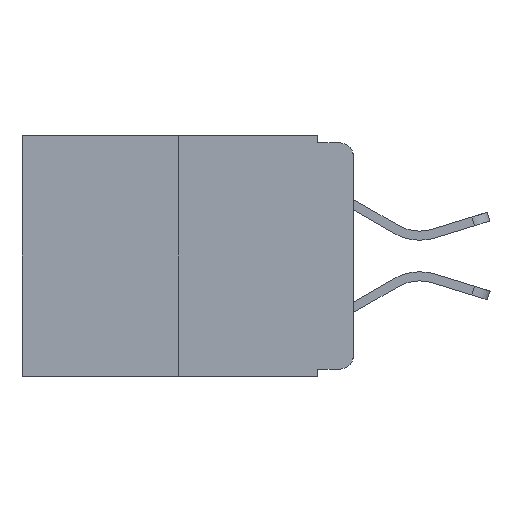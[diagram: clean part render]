
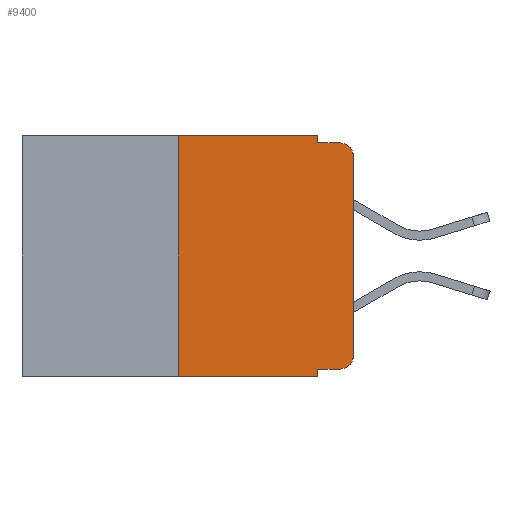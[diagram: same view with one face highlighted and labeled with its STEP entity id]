
A CAD part, left-side view. The second image highlights one B-rep face of the part: STEP entity #9400.
In plain terms, the highlighted planar face has unit normal (-1, 0, 0).
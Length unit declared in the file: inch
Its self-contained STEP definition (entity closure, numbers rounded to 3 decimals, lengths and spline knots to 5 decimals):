
#625 = LINE ( 'NONE', #13521, #10112 ) ;
#638 = EDGE_CURVE ( 'NONE', #16584, #15708, #14473, .T. ) ;
#1058 = ORIENTED_EDGE ( 'NONE', *, *, #5040, .T. ) ;
#1407 = CARTESIAN_POINT ( 'NONE',  ( 0., 0.25, 0. ) ) ;
#1543 = LINE ( 'NONE', #2735, #7409 ) ;
#1629 = ORIENTED_EDGE ( 'NONE', *, *, #3790, .T. ) ;
#2306 = CARTESIAN_POINT ( 'NONE',  ( 0., 0.051, 0. ) ) ;
#2574 = CIRCLE ( 'NONE', #13449, 0.02 ) ;
#2659 = ORIENTED_EDGE ( 'NONE', *, *, #20223, .F. ) ;
#2735 = CARTESIAN_POINT ( 'NONE',  ( 0., 0.473, -0.343 ) ) ;
#2738 = EDGE_CURVE ( 'NONE', #10975, #7517, #20059, .T. ) ;
#3047 = DIRECTION ( 'NONE',  ( 0., -1., 0. ) ) ;
#3286 = DIRECTION ( 'NONE',  ( 0., 0., -1. ) ) ;
#3416 = AXIS2_PLACEMENT_3D ( 'NONE', #12860, #17867, #3286 ) ;
#3738 = DIRECTION ( 'NONE',  ( 0., 0., 1. ) ) ;
#3790 = EDGE_CURVE ( 'NONE', #5624, #16306, #1543, .T. ) ;
#4012 = VERTEX_POINT ( 'NONE', #6872 ) ;
#4794 = CARTESIAN_POINT ( 'NONE',  ( 0., 0.051, -0.333 ) ) ;
#5040 = EDGE_CURVE ( 'NONE', #9668, #16584, #625, .T. ) ;
#5222 = VERTEX_POINT ( 'NONE', #7652 ) ;
#5250 = CARTESIAN_POINT ( 'NONE',  ( 0., 0.051, -0.01 ) ) ;
#5541 = ORIENTED_EDGE ( 'NONE', *, *, #6888, .T. ) ;
#5624 = VERTEX_POINT ( 'NONE', #10834 ) ;
#5826 = CARTESIAN_POINT ( 'NONE',  ( 0., 0., -0.313 ) ) ;
#6172 = EDGE_CURVE ( 'NONE', #5222, #15491, #6612, .T. ) ;
#6262 = EDGE_LOOP ( 'NONE', ( #1058, #16163, #14647, #13093, #2659, #13469, #1629, #20280, #6649, #5541 ) ) ;
#6320 = LINE ( 'NONE', #20997, #15250 ) ;
#6612 = LINE ( 'NONE', #11404, #10405 ) ;
#6649 = ORIENTED_EDGE ( 'NONE', *, *, #2738, .T. ) ;
#6872 = CARTESIAN_POINT ( 'NONE',  ( 0., 0.25, 0. ) ) ;
#6888 = EDGE_CURVE ( 'NONE', #7517, #9668, #2574, .T. ) ;
#7093 = EDGE_CURVE ( 'NONE', #5624, #4012, #10799, .T. ) ;
#7277 = CARTESIAN_POINT ( 'NONE',  ( 0., 0.051, -0.333 ) ) ;
#7349 = CARTESIAN_POINT ( 'NONE',  ( 0., 0.051, -0.343 ) ) ;
#7409 = VECTOR ( 'NONE', #3047, 39.37008 ) ;
#7517 = VERTEX_POINT ( 'NONE', #20351 ) ;
#7615 = LINE ( 'NONE', #2306, #19256 ) ;
#7652 = CARTESIAN_POINT ( 'NONE',  ( 0., 0.051, 0. ) ) ;
#8524 = EDGE_CURVE ( 'NONE', #15491, #15708, #10046, .T. ) ;
#9400 = ADVANCED_FACE ( 'NONE', ( #11179 ), #19464, .F. ) ;
#9668 = VERTEX_POINT ( 'NONE', #5826 ) ;
#9707 = DIRECTION ( 'NONE',  ( 0., 0., -1. ) ) ;
#10046 = LINE ( 'NONE', #5250, #10790 ) ;
#10112 = VECTOR ( 'NONE', #3738, 39.37008 ) ;
#10157 = DIRECTION ( 'NONE',  ( 0., -1., 0. ) ) ;
#10405 = VECTOR ( 'NONE', #9707, 39.37008 ) ;
#10790 = VECTOR ( 'NONE', #10157, 39.37008 ) ;
#10799 = LINE ( 'NONE', #1407, #11808 ) ;
#10834 = CARTESIAN_POINT ( 'NONE',  ( 0., 0.25, -0.343 ) ) ;
#10975 = VERTEX_POINT ( 'NONE', #4794 ) ;
#11179 = FACE_OUTER_BOUND ( 'NONE', #6262, .T. ) ;
#11404 = CARTESIAN_POINT ( 'NONE',  ( 0., 0.051, 0. ) ) ;
#11808 = VECTOR ( 'NONE', #17500, 39.37008 ) ;
#12276 = DIRECTION ( 'NONE',  ( -1., 0., 0. ) ) ;
#12368 = CARTESIAN_POINT ( 'NONE',  ( 0., 0.02, -0.03 ) ) ;
#12860 = CARTESIAN_POINT ( 'NONE',  ( 0., 0.473, 0. ) ) ;
#13093 = ORIENTED_EDGE ( 'NONE', *, *, #6172, .F. ) ;
#13449 = AXIS2_PLACEMENT_3D ( 'NONE', #20161, #12276, #20374 ) ;
#13469 = ORIENTED_EDGE ( 'NONE', *, *, #7093, .F. ) ;
#13521 = CARTESIAN_POINT ( 'NONE',  ( 0., 0., 0. ) ) ;
#13761 = DIRECTION ( 'NONE',  ( 0., -1., 0. ) ) ;
#14026 = CARTESIAN_POINT ( 'NONE',  ( 0., 0.02, -0.01 ) ) ;
#14473 = CIRCLE ( 'NONE', #20254, 0.02 ) ;
#14647 = ORIENTED_EDGE ( 'NONE', *, *, #8524, .F. ) ;
#15250 = VECTOR ( 'NONE', #17397, 39.37008 ) ;
#15491 = VERTEX_POINT ( 'NONE', #16400 ) ;
#15708 = VERTEX_POINT ( 'NONE', #14026 ) ;
#16163 = ORIENTED_EDGE ( 'NONE', *, *, #638, .T. ) ;
#16306 = VERTEX_POINT ( 'NONE', #7349 ) ;
#16400 = CARTESIAN_POINT ( 'NONE',  ( 0., 0.051, -0.01 ) ) ;
#16584 = VERTEX_POINT ( 'NONE', #18401 ) ;
#17003 = DIRECTION ( 'NONE',  ( 0., 0., -1. ) ) ;
#17283 = EDGE_CURVE ( 'NONE', #10975, #16306, #7615, .T. ) ;
#17397 = DIRECTION ( 'NONE',  ( 0., -1., 0. ) ) ;
#17500 = DIRECTION ( 'NONE',  ( 0., 0., 1. ) ) ;
#17867 = DIRECTION ( 'NONE',  ( 1., 0., 0. ) ) ;
#18401 = CARTESIAN_POINT ( 'NONE',  ( 0., 0., -0.03 ) ) ;
#18808 = VECTOR ( 'NONE', #13761, 39.37008 ) ;
#19068 = DIRECTION ( 'NONE',  ( -1., 0., 0. ) ) ;
#19256 = VECTOR ( 'NONE', #17003, 39.37008 ) ;
#19464 = PLANE ( 'NONE',  #3416 ) ;
#20059 = LINE ( 'NONE', #7277, #18808 ) ;
#20161 = CARTESIAN_POINT ( 'NONE',  ( 0., 0.02, -0.313 ) ) ;
#20223 = EDGE_CURVE ( 'NONE', #4012, #5222, #6320, .T. ) ;
#20254 = AXIS2_PLACEMENT_3D ( 'NONE', #12368, #19068, #20778 ) ;
#20280 = ORIENTED_EDGE ( 'NONE', *, *, #17283, .F. ) ;
#20351 = CARTESIAN_POINT ( 'NONE',  ( 0., 0.02, -0.333 ) ) ;
#20374 = DIRECTION ( 'NONE',  ( 0., 0., -1. ) ) ;
#20778 = DIRECTION ( 'NONE',  ( 0., 0., -1. ) ) ;
#20997 = CARTESIAN_POINT ( 'NONE',  ( 0., 0.473, 0. ) ) ;
